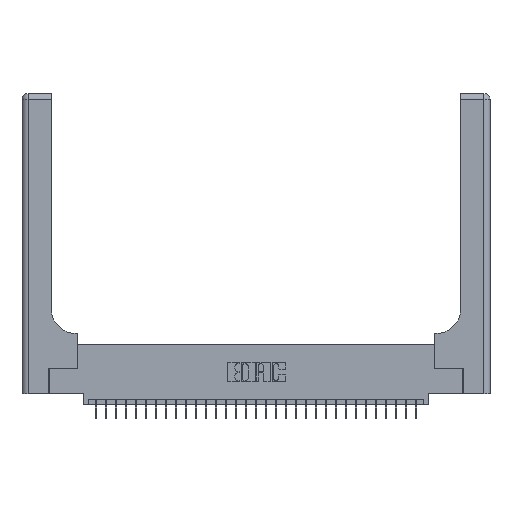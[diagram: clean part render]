
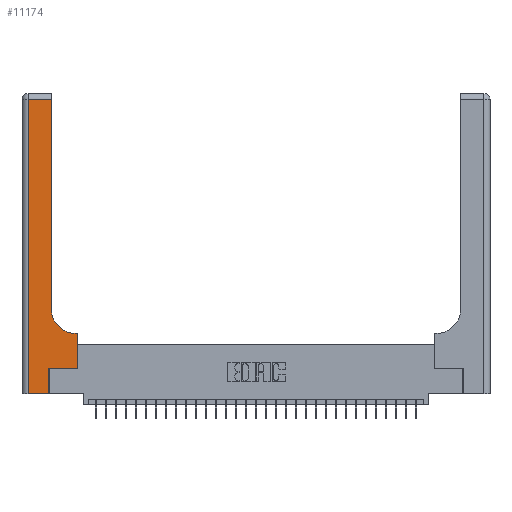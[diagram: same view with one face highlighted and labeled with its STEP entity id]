
A CAD part, top view. The second image highlights one B-rep face of the part: STEP entity #11174.
In plain terms, the highlighted planar face has unit normal (0, 0, 1).
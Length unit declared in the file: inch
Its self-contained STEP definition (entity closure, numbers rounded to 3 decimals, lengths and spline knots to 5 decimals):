
#70 = DIRECTION ( 'NONE',  ( 1., 0., 0. ) ) ;
#130 = CARTESIAN_POINT ( 'NONE',  ( 0.5415, 0.6, 0.37 ) ) ;
#341 = DIRECTION ( 'NONE',  ( 0., 1., 0. ) ) ;
#515 = EDGE_CURVE ( 'NONE', #25479, #17203, #8395, .T. ) ;
#1102 = EDGE_CURVE ( 'NONE', #10869, #25479, #15349, .T. ) ;
#1511 = DIRECTION ( 'NONE',  ( 0., 0., -1. ) ) ;
#2621 = VECTOR ( 'NONE', #70, 39.37008 ) ;
#2705 = DIRECTION ( 'NONE',  ( 0., 1., 0. ) ) ;
#3052 = CARTESIAN_POINT ( 'NONE',  ( 0.2915, 2.94, 0.37 ) ) ;
#3872 = ORIENTED_EDGE ( 'NONE', *, *, #1102, .T. ) ;
#3880 = EDGE_CURVE ( 'NONE', #13065, #27111, #25619, .T. ) ;
#4518 = LINE ( 'NONE', #9604, #12586 ) ;
#5012 = CARTESIAN_POINT ( 'NONE',  ( 0.2915, 3., 0.37 ) ) ;
#5721 = VECTOR ( 'NONE', #29903, 39.37008 ) ;
#6304 = ORIENTED_EDGE ( 'NONE', *, *, #12328, .T. ) ;
#6622 = DIRECTION ( 'NONE',  ( 1., 0., 0. ) ) ;
#6711 = VERTEX_POINT ( 'NONE', #3052 ) ;
#6719 = DIRECTION ( 'NONE',  ( 1., 0., 0. ) ) ;
#7362 = ORIENTED_EDGE ( 'NONE', *, *, #9532, .T. ) ;
#7676 = VECTOR ( 'NONE', #6719, 39.37008 ) ;
#8395 = LINE ( 'NONE', #18446, #28897 ) ;
#8441 = ORIENTED_EDGE ( 'NONE', *, *, #29583, .T. ) ;
#9532 = EDGE_CURVE ( 'NONE', #14056, #6711, #32193, .T. ) ;
#9604 = CARTESIAN_POINT ( 'NONE',  ( 0., 2.94, 0.37 ) ) ;
#9990 = ORIENTED_EDGE ( 'NONE', *, *, #18129, .T. ) ;
#10869 = VERTEX_POINT ( 'NONE', #17528 ) ;
#10922 = DIRECTION ( 'NONE',  ( 0., 1., 0. ) ) ;
#11174 = ADVANCED_FACE ( 'NONE', ( #31991 ), #29053, .F. ) ;
#11463 = CARTESIAN_POINT ( 'NONE',  ( 0.269, 0., 0.37 ) ) ;
#11832 = AXIS2_PLACEMENT_3D ( 'NONE', #31835, #14504, #26426 ) ;
#12328 = EDGE_CURVE ( 'NONE', #17203, #13065, #13522, .T. ) ;
#12583 = CARTESIAN_POINT ( 'NONE',  ( 0., 0., 0.37 ) ) ;
#12586 = VECTOR ( 'NONE', #27418, 39.37008 ) ;
#13065 = VERTEX_POINT ( 'NONE', #20023 ) ;
#13522 = LINE ( 'NONE', #21104, #7676 ) ;
#14056 = VERTEX_POINT ( 'NONE', #21593 ) ;
#14504 = DIRECTION ( 'NONE',  ( 0., 0., -1. ) ) ;
#15349 = LINE ( 'NONE', #12583, #2621 ) ;
#15415 = VECTOR ( 'NONE', #2705, 39.37008 ) ;
#16110 = EDGE_CURVE ( 'NONE', #27111, #25036, #22150, .T. ) ;
#16384 = AXIS2_PLACEMENT_3D ( 'NONE', #21766, #1511, #6622 ) ;
#16585 = ORIENTED_EDGE ( 'NONE', *, *, #515, .T. ) ;
#17203 = VERTEX_POINT ( 'NONE', #29498 ) ;
#17528 = CARTESIAN_POINT ( 'NONE',  ( 0.06, 0., 0.37 ) ) ;
#18129 = EDGE_CURVE ( 'NONE', #6711, #22137, #4518, .T. ) ;
#18446 = CARTESIAN_POINT ( 'NONE',  ( 0.269, 0., 0.37 ) ) ;
#18685 = CARTESIAN_POINT ( 'NONE',  ( 0.06, 3., 0.37 ) ) ;
#19336 = LINE ( 'NONE', #18685, #29508 ) ;
#20023 = CARTESIAN_POINT ( 'NONE',  ( 0.5585, 0.25, 0.37 ) ) ;
#20678 = ORIENTED_EDGE ( 'NONE', *, *, #3880, .T. ) ;
#21104 = CARTESIAN_POINT ( 'NONE',  ( 0.269, 0.25, 0.37 ) ) ;
#21593 = CARTESIAN_POINT ( 'NONE',  ( 0.2915, 0.85, 0.37 ) ) ;
#21639 = CARTESIAN_POINT ( 'NONE',  ( 0.5585, 0.6, 0.37 ) ) ;
#21766 = CARTESIAN_POINT ( 'NONE',  ( 0.5415, 0.85, 0.37 ) ) ;
#21988 = EDGE_LOOP ( 'NONE', ( #7362, #9990, #24936, #3872, #16585, #6304, #20678, #26153, #8441 ) ) ;
#22063 = CARTESIAN_POINT ( 'NONE',  ( 0.06, 2.94, 0.37 ) ) ;
#22137 = VERTEX_POINT ( 'NONE', #22063 ) ;
#22150 = LINE ( 'NONE', #31876, #5721 ) ;
#22195 = VECTOR ( 'NONE', #10922, 39.37008 ) ;
#23309 = CARTESIAN_POINT ( 'NONE',  ( 0.5585, 0.25, 0.37 ) ) ;
#23798 = DIRECTION ( 'NONE',  ( 0., -1., 0. ) ) ;
#24936 = ORIENTED_EDGE ( 'NONE', *, *, #27024, .T. ) ;
#25036 = VERTEX_POINT ( 'NONE', #130 ) ;
#25479 = VERTEX_POINT ( 'NONE', #11463 ) ;
#25619 = LINE ( 'NONE', #23309, #22195 ) ;
#26153 = ORIENTED_EDGE ( 'NONE', *, *, #16110, .T. ) ;
#26426 = DIRECTION ( 'NONE',  ( -1., 0., 0. ) ) ;
#27024 = EDGE_CURVE ( 'NONE', #22137, #10869, #19336, .T. ) ;
#27111 = VERTEX_POINT ( 'NONE', #21639 ) ;
#27418 = DIRECTION ( 'NONE',  ( -1., 0., 0. ) ) ;
#28897 = VECTOR ( 'NONE', #341, 39.37008 ) ;
#29053 = PLANE ( 'NONE',  #11832 ) ;
#29498 = CARTESIAN_POINT ( 'NONE',  ( 0.269, 0.25, 0.37 ) ) ;
#29508 = VECTOR ( 'NONE', #23798, 39.37008 ) ;
#29583 = EDGE_CURVE ( 'NONE', #25036, #14056, #31655, .T. ) ;
#29903 = DIRECTION ( 'NONE',  ( -1., 0., 0. ) ) ;
#31655 = CIRCLE ( 'NONE', #16384, 0.25 ) ;
#31835 = CARTESIAN_POINT ( 'NONE',  ( 0., 3., 0.37 ) ) ;
#31876 = CARTESIAN_POINT ( 'NONE',  ( 0.2915, 0.6, 0.37 ) ) ;
#31991 = FACE_OUTER_BOUND ( 'NONE', #21988, .T. ) ;
#32193 = LINE ( 'NONE', #5012, #15415 ) ;
